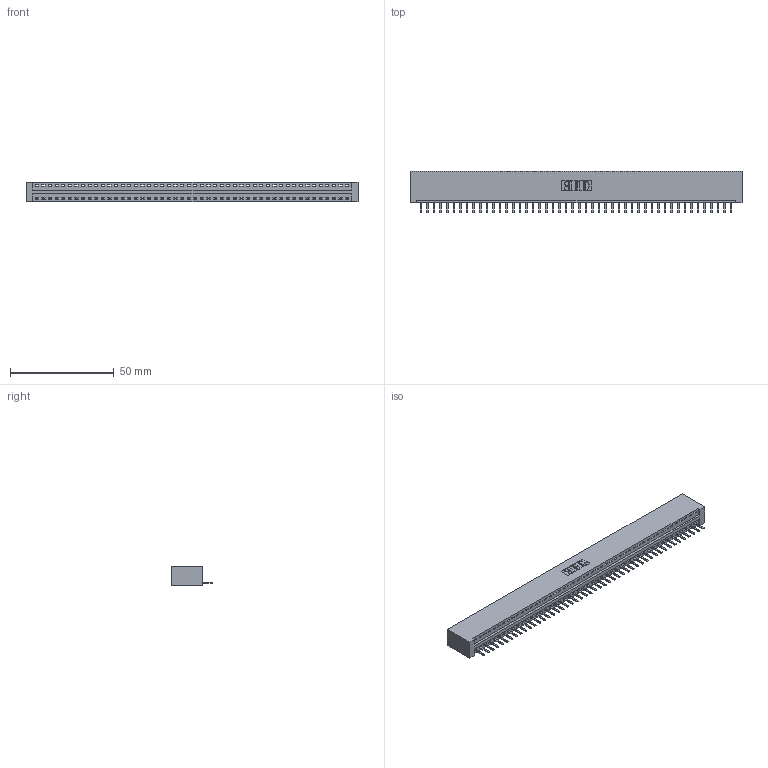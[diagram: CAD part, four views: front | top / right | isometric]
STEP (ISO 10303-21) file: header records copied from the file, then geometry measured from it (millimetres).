
FILE_DESCRIPTION (( 'STEP AP203' ), '1' );
FILE_NAME ('396-048-520-101.STEP', '2018-09-07T11:32:34', ( '' ), ( '' ), 'SwSTEP 2.0', 'SolidWorks 2016', '' );
FILE_SCHEMA (( 'CONFIG_CONTROL_DESIGN' ));
Length unit declared in the file: inch
Products named in the file (3): 346 Part_No Mounting Lugs; 345-292-001_345-293-120; 396-048-520-101
Assembly tree (49 placements, depth 2):
  396-048-520-101
    346 Part_No Mounting Lugs
    345-292-001_345-293-120  x48
Bounding box: 159.64 x 20.02 x 9.4 mm (x, y, z)
Volume: 15733.7 mm3; surface area: 19344 mm2
Topology: 49 solids, 49 shells, 3090 faces, 9137 edges, 5962 vertices
Faces by surface type: plane 2088, cylinder 1002
Entity records: 28819 total; most frequent: CARTESIAN_POINT 4956, ORIENTED_EDGE 4926, DIRECTION 4347, EDGE_CURVE 2463, LINE 2143, VECTOR 2143, VERTEX_POINT 1638, AXIS2_PLACEMENT_3D 1102
